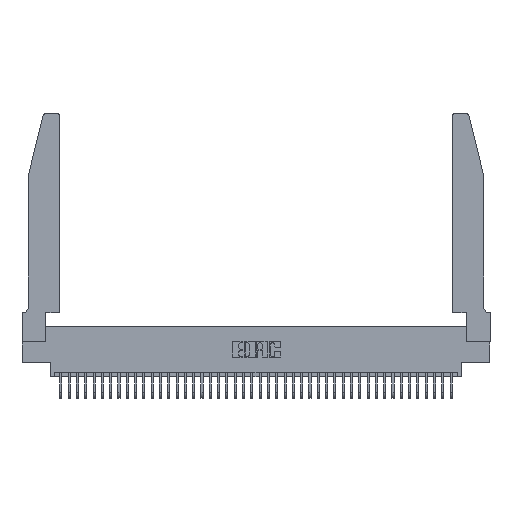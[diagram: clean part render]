
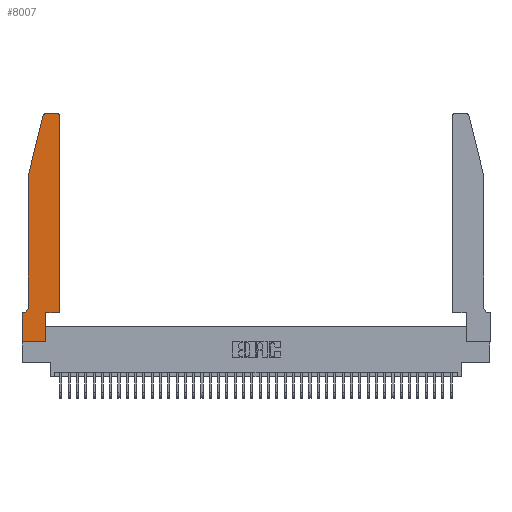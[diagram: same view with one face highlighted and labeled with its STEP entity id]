
A CAD part, top view. The second image highlights one B-rep face of the part: STEP entity #8007.
In plain terms, the highlighted planar face has unit normal (0, 0, 1).
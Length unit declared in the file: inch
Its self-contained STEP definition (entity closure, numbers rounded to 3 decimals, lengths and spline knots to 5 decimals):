
#1022 = ORIENTED_EDGE ( 'NONE', *, *, #28429, .T. ) ;
#1046 = DIRECTION ( 'NONE',  ( -1., 0., 0. ) ) ;
#1266 = CARTESIAN_POINT ( 'NONE',  ( 0.4505, 0.35, 0.37 ) ) ;
#1370 = ORIENTED_EDGE ( 'NONE', *, *, #22321, .T. ) ;
#1442 = CARTESIAN_POINT ( 'NONE',  ( 0., 0.35, 0.37 ) ) ;
#1569 = CARTESIAN_POINT ( 'NONE',  ( 0., 0., 0.37 ) ) ;
#2049 = VERTEX_POINT ( 'NONE', #28948 ) ;
#2415 = VECTOR ( 'NONE', #16587, 39.37008 ) ;
#2450 = CIRCLE ( 'NONE', #16905, 0.03 ) ;
#2482 = ORIENTED_EDGE ( 'NONE', *, *, #5464, .T. ) ;
#2622 = DIRECTION ( 'NONE',  ( 1., 0., 0. ) ) ;
#2745 = DIRECTION ( 'NONE',  ( 0., -1., 0. ) ) ;
#5228 = DIRECTION ( 'NONE',  ( 1., 0., 0. ) ) ;
#5442 = VERTEX_POINT ( 'NONE', #11162 ) ;
#5464 = EDGE_CURVE ( 'NONE', #39031, #10225, #35922, .T. ) ;
#5582 = LINE ( 'NONE', #29681, #30276 ) ;
#5602 = DIRECTION ( 'NONE',  ( -1., 0., 0. ) ) ;
#5749 = CARTESIAN_POINT ( 'NONE',  ( 0.284, 2.75, 0.37 ) ) ;
#6030 = ORIENTED_EDGE ( 'NONE', *, *, #14161, .T. ) ;
#6797 = AXIS2_PLACEMENT_3D ( 'NONE', #27211, #7125, #30580 ) ;
#7125 = DIRECTION ( 'NONE',  ( 0., 0., 1. ) ) ;
#7387 = VERTEX_POINT ( 'NONE', #1442 ) ;
#8007 = ADVANCED_FACE ( 'NONE', ( #19101 ), #18646, .T. ) ;
#9673 = CARTESIAN_POINT ( 'NONE',  ( 0.0755, 2., 0.37 ) ) ;
#10225 = VERTEX_POINT ( 'NONE', #27678 ) ;
#10892 = CARTESIAN_POINT ( 'NONE',  ( 0.2865, 0.35, 0.37 ) ) ;
#10948 = VECTOR ( 'NONE', #16208, 39.37008 ) ;
#11000 = VERTEX_POINT ( 'NONE', #1569 ) ;
#11020 = VERTEX_POINT ( 'NONE', #38510 ) ;
#11162 = CARTESIAN_POINT ( 'NONE',  ( 0.0755, 0.42, 0.37 ) ) ;
#11443 = CARTESIAN_POINT ( 'NONE',  ( 0.4505, 0.35, 0.37 ) ) ;
#11501 = LINE ( 'NONE', #23184, #2415 ) ;
#11847 = CARTESIAN_POINT ( 'NONE',  ( 0.25487, 2.72718, 0.37 ) ) ;
#12173 = EDGE_CURVE ( 'NONE', #5442, #11020, #35123, .T. ) ;
#12771 = ORIENTED_EDGE ( 'NONE', *, *, #12173, .T. ) ;
#12994 = EDGE_CURVE ( 'NONE', #10225, #2049, #2450, .T. ) ;
#13181 = DIRECTION ( 'NONE',  ( 1., 0., 0. ) ) ;
#14161 = EDGE_CURVE ( 'NONE', #42056, #41910, #19277, .T. ) ;
#14370 = ORIENTED_EDGE ( 'NONE', *, *, #17492, .T. ) ;
#15126 = LINE ( 'NONE', #32466, #39610 ) ;
#15358 = LINE ( 'NONE', #27854, #32127 ) ;
#16208 = DIRECTION ( 'NONE',  ( -0.239, -0.971, 0. ) ) ;
#16587 = DIRECTION ( 'NONE',  ( 1., 0., 0. ) ) ;
#16905 = AXIS2_PLACEMENT_3D ( 'NONE', #42722, #22811, #2622 ) ;
#17492 = EDGE_CURVE ( 'NONE', #38748, #42998, #15358, .T. ) ;
#18022 = LINE ( 'NONE', #24373, #34737 ) ;
#18068 = ORIENTED_EDGE ( 'NONE', *, *, #25406, .T. ) ;
#18540 = ORIENTED_EDGE ( 'NONE', *, *, #35677, .T. ) ;
#18646 = PLANE ( 'NONE',  #42103 ) ;
#19101 = FACE_OUTER_BOUND ( 'NONE', #19334, .T. ) ;
#19277 = CIRCLE ( 'NONE', #6797, 0.03 ) ;
#19334 = EDGE_LOOP ( 'NONE', ( #1022, #6030, #34853, #35758, #12771, #1370, #18540, #18068, #14370, #41443, #2482, #19421 ) ) ;
#19421 = ORIENTED_EDGE ( 'NONE', *, *, #12994, .T. ) ;
#21284 = DIRECTION ( 'NONE',  ( 0., 0., -1. ) ) ;
#21633 = AXIS2_PLACEMENT_3D ( 'NONE', #41216, #21284, #1046 ) ;
#22321 = EDGE_CURVE ( 'NONE', #11020, #7387, #15126, .T. ) ;
#22429 = EDGE_CURVE ( 'NONE', #41910, #23433, #28724, .T. ) ;
#22808 = CARTESIAN_POINT ( 'NONE',  ( 0.2865, 0., 0.37 ) ) ;
#22811 = DIRECTION ( 'NONE',  ( 0., 0., 1. ) ) ;
#22929 = CARTESIAN_POINT ( 'NONE',  ( 0.0755, 2., 0.37 ) ) ;
#23184 = CARTESIAN_POINT ( 'NONE',  ( 0.4505, 0.35, 0.37 ) ) ;
#23433 = VERTEX_POINT ( 'NONE', #9673 ) ;
#24373 = CARTESIAN_POINT ( 'NONE',  ( 0.2605, 2.75, 0.37 ) ) ;
#24729 = EDGE_CURVE ( 'NONE', #42998, #39031, #11501, .T. ) ;
#25366 = DIRECTION ( 'NONE',  ( 0., 0., 1. ) ) ;
#25406 = EDGE_CURVE ( 'NONE', #11000, #38748, #38102, .T. ) ;
#26481 = LINE ( 'NONE', #27477, #34333 ) ;
#27107 = VECTOR ( 'NONE', #34814, 39.37008 ) ;
#27211 = CARTESIAN_POINT ( 'NONE',  ( 0.284, 2.72, 0.37 ) ) ;
#27477 = CARTESIAN_POINT ( 'NONE',  ( 0.0755, 2., 0.37 ) ) ;
#27678 = CARTESIAN_POINT ( 'NONE',  ( 0.4505, 2.72, 0.37 ) ) ;
#27854 = CARTESIAN_POINT ( 'NONE',  ( 0.2865, 0.35, 0.37 ) ) ;
#28429 = EDGE_CURVE ( 'NONE', #2049, #42056, #18022, .T. ) ;
#28724 = LINE ( 'NONE', #22929, #10948 ) ;
#28948 = CARTESIAN_POINT ( 'NONE',  ( 0.4205, 2.75, 0.37 ) ) ;
#29681 = CARTESIAN_POINT ( 'NONE',  ( 0., 0., 0.37 ) ) ;
#30276 = VECTOR ( 'NONE', #2745, 39.37008 ) ;
#30368 = VECTOR ( 'NONE', #13181, 39.37008 ) ;
#30580 = DIRECTION ( 'NONE',  ( 1., 0., 0. ) ) ;
#30834 = DIRECTION ( 'NONE',  ( 0., -1., 0. ) ) ;
#31113 = DIRECTION ( 'NONE',  ( -1., 0., 0. ) ) ;
#31215 = DIRECTION ( 'NONE',  ( 0., 1., 0. ) ) ;
#32127 = VECTOR ( 'NONE', #31215, 39.37008 ) ;
#32466 = CARTESIAN_POINT ( 'NONE',  ( 0.0755, 0.35, 0.37 ) ) ;
#33247 = CARTESIAN_POINT ( 'NONE',  ( 0., 0., 0.37 ) ) ;
#34333 = VECTOR ( 'NONE', #30834, 39.37008 ) ;
#34737 = VECTOR ( 'NONE', #31113, 39.37008 ) ;
#34814 = DIRECTION ( 'NONE',  ( 0., 1., 0. ) ) ;
#34853 = ORIENTED_EDGE ( 'NONE', *, *, #22429, .T. ) ;
#35123 = CIRCLE ( 'NONE', #21633, 0.07 ) ;
#35677 = EDGE_CURVE ( 'NONE', #7387, #11000, #5582, .T. ) ;
#35758 = ORIENTED_EDGE ( 'NONE', *, *, #39568, .T. ) ;
#35922 = LINE ( 'NONE', #11443, #27107 ) ;
#38102 = LINE ( 'NONE', #33247, #30368 ) ;
#38510 = CARTESIAN_POINT ( 'NONE',  ( 0.0055, 0.35, 0.37 ) ) ;
#38748 = VERTEX_POINT ( 'NONE', #22808 ) ;
#39031 = VERTEX_POINT ( 'NONE', #1266 ) ;
#39568 = EDGE_CURVE ( 'NONE', #23433, #5442, #26481, .T. ) ;
#39610 = VECTOR ( 'NONE', #5602, 39.37008 ) ;
#41216 = CARTESIAN_POINT ( 'NONE',  ( 0.0055, 0.42, 0.37 ) ) ;
#41443 = ORIENTED_EDGE ( 'NONE', *, *, #24729, .T. ) ;
#41899 = CARTESIAN_POINT ( 'NONE',  ( 0., 0.35, 0.37 ) ) ;
#41910 = VERTEX_POINT ( 'NONE', #11847 ) ;
#42056 = VERTEX_POINT ( 'NONE', #5749 ) ;
#42103 = AXIS2_PLACEMENT_3D ( 'NONE', #41899, #25366, #5228 ) ;
#42722 = CARTESIAN_POINT ( 'NONE',  ( 0.4205, 2.72, 0.37 ) ) ;
#42998 = VERTEX_POINT ( 'NONE', #10892 ) ;
